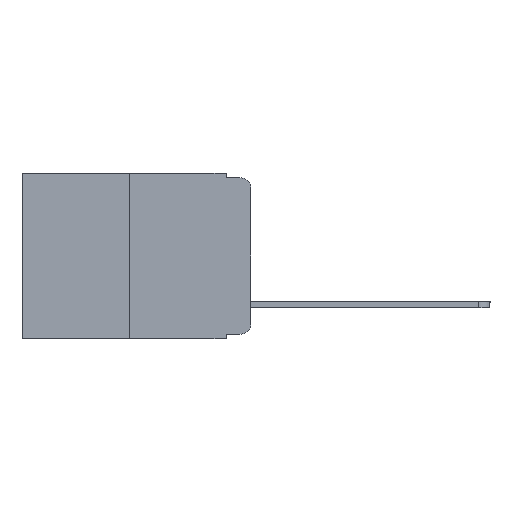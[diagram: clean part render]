
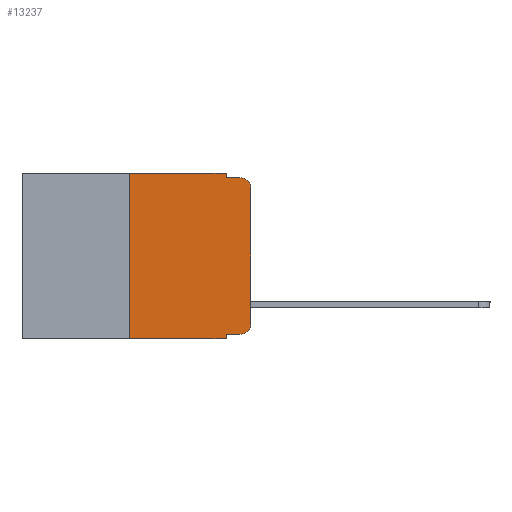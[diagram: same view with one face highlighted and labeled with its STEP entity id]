
A CAD part, left-side view. The second image highlights one B-rep face of the part: STEP entity #13237.
In plain terms, the highlighted planar face has unit normal (-1, 0, 0).
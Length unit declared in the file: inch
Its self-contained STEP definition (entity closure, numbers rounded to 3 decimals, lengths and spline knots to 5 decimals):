
#246 = VERTEX_POINT ( 'NONE', #17131 ) ;
#661 = EDGE_CURVE ( 'NONE', #18636, #5073, #4034, .T. ) ;
#792 = AXIS2_PLACEMENT_3D ( 'NONE', #17068, #7782, #4901 ) ;
#863 = DIRECTION ( 'NONE',  ( 0., -1., 0. ) ) ;
#1117 = DIRECTION ( 'NONE',  ( 0., 0., 1. ) ) ;
#1253 = VERTEX_POINT ( 'NONE', #17657 ) ;
#1463 = LINE ( 'NONE', #12261, #2983 ) ;
#1530 = EDGE_LOOP ( 'NONE', ( #3717, #18888, #6770, #13757, #3614, #9653, #7922, #11135, #18547, #10690 ) ) ;
#1736 = VECTOR ( 'NONE', #1117, 39.37008 ) ;
#2117 = EDGE_CURVE ( 'NONE', #15515, #246, #1463, .T. ) ;
#2375 = EDGE_CURVE ( 'NONE', #13017, #17732, #16731, .T. ) ;
#2524 = CARTESIAN_POINT ( 'NONE',  ( 0., 0.473, 0. ) ) ;
#2658 = LINE ( 'NONE', #3054, #11382 ) ;
#2983 = VECTOR ( 'NONE', #7420, 39.37008 ) ;
#3014 = EDGE_CURVE ( 'NONE', #5537, #9550, #8218, .T. ) ;
#3054 = CARTESIAN_POINT ( 'NONE',  ( 0., 0.051, 0. ) ) ;
#3360 = LINE ( 'NONE', #5055, #6676 ) ;
#3614 = ORIENTED_EDGE ( 'NONE', *, *, #2117, .F. ) ;
#3717 = ORIENTED_EDGE ( 'NONE', *, *, #15331, .T. ) ;
#4034 = LINE ( 'NONE', #14229, #18742 ) ;
#4153 = DIRECTION ( 'NONE',  ( 0., 0., -1. ) ) ;
#4901 = DIRECTION ( 'NONE',  ( 0., 0., -1. ) ) ;
#5055 = CARTESIAN_POINT ( 'NONE',  ( 0., 0.051, 0. ) ) ;
#5073 = VERTEX_POINT ( 'NONE', #9464 ) ;
#5154 = CARTESIAN_POINT ( 'NONE',  ( 0., 0.051, -0.01 ) ) ;
#5260 = DIRECTION ( 'NONE',  ( 0., 0., -1. ) ) ;
#5404 = DIRECTION ( 'NONE',  ( 1., 0., 0. ) ) ;
#5537 = VERTEX_POINT ( 'NONE', #8043 ) ;
#5965 = CARTESIAN_POINT ( 'NONE',  ( 0., 0., -0.03 ) ) ;
#6669 = LINE ( 'NONE', #6756, #10370 ) ;
#6676 = VECTOR ( 'NONE', #10988, 39.37008 ) ;
#6756 = CARTESIAN_POINT ( 'NONE',  ( 0., 0.25, 0. ) ) ;
#6770 = ORIENTED_EDGE ( 'NONE', *, *, #2375, .F. ) ;
#7150 = VECTOR ( 'NONE', #14319, 39.37008 ) ;
#7249 = AXIS2_PLACEMENT_3D ( 'NONE', #12686, #12879, #5260 ) ;
#7380 = CARTESIAN_POINT ( 'NONE',  ( 0., 0.051, -0.343 ) ) ;
#7420 = DIRECTION ( 'NONE',  ( 0., -1., 0. ) ) ;
#7782 = DIRECTION ( 'NONE',  ( -1., 0., 0. ) ) ;
#7922 = ORIENTED_EDGE ( 'NONE', *, *, #3014, .T. ) ;
#8043 = CARTESIAN_POINT ( 'NONE',  ( 0., 0.25, -0.343 ) ) ;
#8218 = LINE ( 'NONE', #19050, #7150 ) ;
#8663 = PLANE ( 'NONE',  #14120 ) ;
#8865 = CARTESIAN_POINT ( 'NONE',  ( 0., 0., 0. ) ) ;
#9060 = EDGE_CURVE ( 'NONE', #18636, #9550, #2658, .T. ) ;
#9450 = CARTESIAN_POINT ( 'NONE',  ( 0., 0.25, 0. ) ) ;
#9464 = CARTESIAN_POINT ( 'NONE',  ( 0., 0.02, -0.333 ) ) ;
#9550 = VERTEX_POINT ( 'NONE', #7380 ) ;
#9641 = DIRECTION ( 'NONE',  ( 0., 0., 1. ) ) ;
#9653 = ORIENTED_EDGE ( 'NONE', *, *, #16826, .F. ) ;
#10318 = EDGE_CURVE ( 'NONE', #246, #13017, #3360, .T. ) ;
#10370 = VECTOR ( 'NONE', #9641, 39.37008 ) ;
#10690 = ORIENTED_EDGE ( 'NONE', *, *, #18436, .T. ) ;
#10988 = DIRECTION ( 'NONE',  ( 0., 0., -1. ) ) ;
#11135 = ORIENTED_EDGE ( 'NONE', *, *, #9060, .F. ) ;
#11382 = VECTOR ( 'NONE', #4153, 39.37008 ) ;
#12015 = DIRECTION ( 'NONE',  ( 0., -1., 0. ) ) ;
#12183 = CIRCLE ( 'NONE', #792, 0.02 ) ;
#12261 = CARTESIAN_POINT ( 'NONE',  ( 0., 0.473, 0. ) ) ;
#12686 = CARTESIAN_POINT ( 'NONE',  ( 0., 0.02, -0.313 ) ) ;
#12879 = DIRECTION ( 'NONE',  ( -1., 0., 0. ) ) ;
#13017 = VERTEX_POINT ( 'NONE', #15376 ) ;
#13103 = FACE_OUTER_BOUND ( 'NONE', #1530, .T. ) ;
#13237 = ADVANCED_FACE ( 'NONE', ( #13103 ), #8663, .F. ) ;
#13757 = ORIENTED_EDGE ( 'NONE', *, *, #10318, .F. ) ;
#14120 = AXIS2_PLACEMENT_3D ( 'NONE', #2524, #5404, #17448 ) ;
#14229 = CARTESIAN_POINT ( 'NONE',  ( 0., 0.051, -0.333 ) ) ;
#14319 = DIRECTION ( 'NONE',  ( 0., -1., 0. ) ) ;
#14528 = CARTESIAN_POINT ( 'NONE',  ( 0., 0.02, -0.01 ) ) ;
#15072 = EDGE_CURVE ( 'NONE', #18189, #17732, #12183, .T. ) ;
#15331 = EDGE_CURVE ( 'NONE', #1253, #18189, #17652, .T. ) ;
#15376 = CARTESIAN_POINT ( 'NONE',  ( 0., 0.051, -0.01 ) ) ;
#15515 = VERTEX_POINT ( 'NONE', #9450 ) ;
#16066 = CIRCLE ( 'NONE', #7249, 0.02 ) ;
#16731 = LINE ( 'NONE', #5154, #19438 ) ;
#16826 = EDGE_CURVE ( 'NONE', #5537, #15515, #6669, .T. ) ;
#17068 = CARTESIAN_POINT ( 'NONE',  ( 0., 0.02, -0.03 ) ) ;
#17091 = CARTESIAN_POINT ( 'NONE',  ( 0., 0.051, -0.333 ) ) ;
#17131 = CARTESIAN_POINT ( 'NONE',  ( 0., 0.051, 0. ) ) ;
#17448 = DIRECTION ( 'NONE',  ( 0., 0., -1. ) ) ;
#17652 = LINE ( 'NONE', #8865, #1736 ) ;
#17657 = CARTESIAN_POINT ( 'NONE',  ( 0., 0., -0.313 ) ) ;
#17732 = VERTEX_POINT ( 'NONE', #14528 ) ;
#18189 = VERTEX_POINT ( 'NONE', #5965 ) ;
#18436 = EDGE_CURVE ( 'NONE', #5073, #1253, #16066, .T. ) ;
#18547 = ORIENTED_EDGE ( 'NONE', *, *, #661, .T. ) ;
#18636 = VERTEX_POINT ( 'NONE', #17091 ) ;
#18742 = VECTOR ( 'NONE', #863, 39.37008 ) ;
#18888 = ORIENTED_EDGE ( 'NONE', *, *, #15072, .T. ) ;
#19050 = CARTESIAN_POINT ( 'NONE',  ( 0., 0.473, -0.343 ) ) ;
#19438 = VECTOR ( 'NONE', #12015, 39.37008 ) ;
